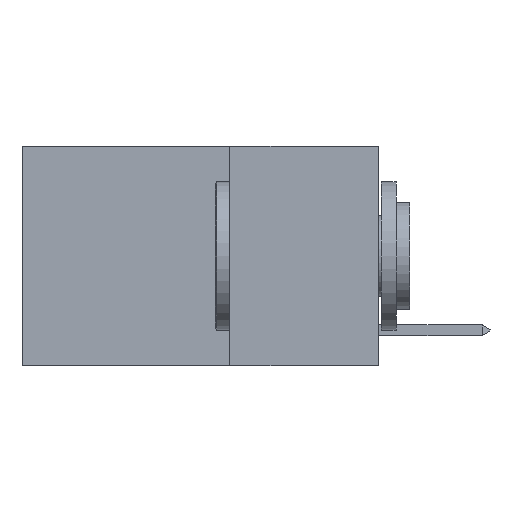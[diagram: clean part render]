
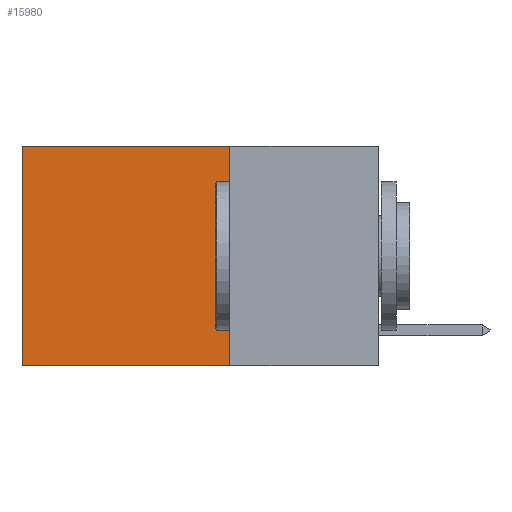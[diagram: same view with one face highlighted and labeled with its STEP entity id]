
A CAD part, left-side view. The second image highlights one B-rep face of the part: STEP entity #15980.
In plain terms, the highlighted planar face has unit normal (-1, 0, 0).
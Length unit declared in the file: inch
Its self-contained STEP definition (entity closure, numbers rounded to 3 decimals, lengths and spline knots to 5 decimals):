
#103 = VERTEX_POINT ( 'NONE', #7865 ) ;
#320 = DIRECTION ( 'NONE',  ( 0., 1., 0. ) ) ;
#1601 = VERTEX_POINT ( 'NONE', #14776 ) ;
#1863 = VECTOR ( 'NONE', #9442, 39.37008 ) ;
#3596 = ORIENTED_EDGE ( 'NONE', *, *, #8124, .F. ) ;
#4403 = DIRECTION ( 'NONE',  ( 1., 0., 0. ) ) ;
#4813 = DIRECTION ( 'NONE',  ( 0., 0., -1. ) ) ;
#5107 = LINE ( 'NONE', #22872, #14592 ) ;
#5369 = VECTOR ( 'NONE', #8780, 39.37008 ) ;
#6881 = CARTESIAN_POINT ( 'NONE',  ( 0.2625, 0.6, 0. ) ) ;
#7543 = CARTESIAN_POINT ( 'NONE',  ( 0.2625, 0.25, -0.37 ) ) ;
#7712 = VECTOR ( 'NONE', #4813, 39.37008 ) ;
#7865 = CARTESIAN_POINT ( 'NONE',  ( 0.2625, 0.25, 0. ) ) ;
#8124 = EDGE_CURVE ( 'NONE', #103, #22553, #13320, .T. ) ;
#8565 = CARTESIAN_POINT ( 'NONE',  ( 0.2625, 0.25, -0.37 ) ) ;
#8780 = DIRECTION ( 'NONE',  ( 0., 0., -1. ) ) ;
#9442 = DIRECTION ( 'NONE',  ( 0., 1., 0. ) ) ;
#10132 = CARTESIAN_POINT ( 'NONE',  ( 0.2625, 0.6, -0.37 ) ) ;
#10267 = EDGE_CURVE ( 'NONE', #22553, #11134, #16996, .T. ) ;
#11134 = VERTEX_POINT ( 'NONE', #10132 ) ;
#11720 = EDGE_CURVE ( 'NONE', #103, #1601, #5107, .T. ) ;
#11969 = PLANE ( 'NONE',  #19096 ) ;
#12262 = ORIENTED_EDGE ( 'NONE', *, *, #10267, .F. ) ;
#12354 = CARTESIAN_POINT ( 'NONE',  ( 0.2625, 0.25, 0. ) ) ;
#13320 = LINE ( 'NONE', #12354, #7712 ) ;
#13786 = ORIENTED_EDGE ( 'NONE', *, *, #11720, .T. ) ;
#13873 = CARTESIAN_POINT ( 'NONE',  ( 0.2625, 0.25, 0. ) ) ;
#14592 = VECTOR ( 'NONE', #320, 39.37008 ) ;
#14776 = CARTESIAN_POINT ( 'NONE',  ( 0.2625, 0.6, 0. ) ) ;
#14848 = LINE ( 'NONE', #6881, #5369 ) ;
#15980 = ADVANCED_FACE ( 'NONE', ( #22633 ), #11969, .F. ) ;
#16996 = LINE ( 'NONE', #7543, #1863 ) ;
#17599 = DIRECTION ( 'NONE',  ( 0., 0., -1. ) ) ;
#19096 = AXIS2_PLACEMENT_3D ( 'NONE', #13873, #4403, #17599 ) ;
#19616 = EDGE_LOOP ( 'NONE', ( #22042, #12262, #3596, #13786 ) ) ;
#21173 = EDGE_CURVE ( 'NONE', #1601, #11134, #14848, .T. ) ;
#22042 = ORIENTED_EDGE ( 'NONE', *, *, #21173, .T. ) ;
#22553 = VERTEX_POINT ( 'NONE', #8565 ) ;
#22633 = FACE_OUTER_BOUND ( 'NONE', #19616, .T. ) ;
#22872 = CARTESIAN_POINT ( 'NONE',  ( 0.2625, 0.25, 0. ) ) ;
